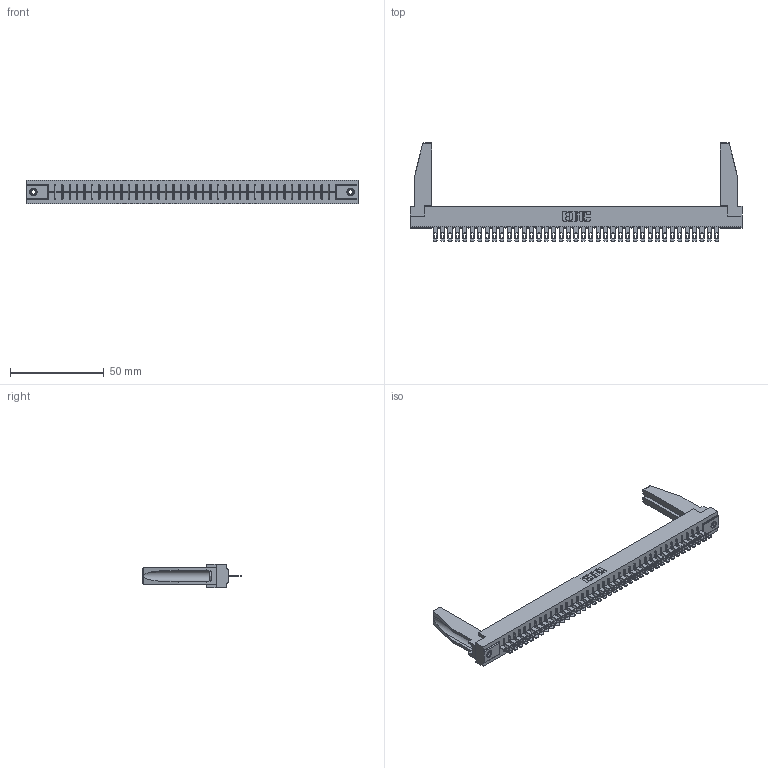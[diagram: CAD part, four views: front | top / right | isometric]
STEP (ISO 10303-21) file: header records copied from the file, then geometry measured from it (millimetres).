
FILE_DESCRIPTION (( 'STEP AP203' ), '1' );
FILE_NAME ('356-039-400-178.STEP', '2020-09-24T00:03:07', ( '' ), ( '' ), 'SwSTEP 2.0', 'SolidWorks 2020', '' );
FILE_SCHEMA (( 'CONFIG_CONTROL_DESIGN' ));
Length unit declared in the file: inch
Products named in the file (5): 306 Part_.156 Dia; 356-039-400-178; 307-220-078; 306-290-001_100; 345-250-001_345-250-001-102
Assembly tree (44 placements, depth 2):
  356-039-400-178
    306 Part_.156 Dia
    306-290-001_100  x39
    345-250-001_345-250-001-102  x2
    307-220-078  x2
Bounding box: 177.55 x 52.91 x 12.7 mm (x, y, z)
Volume: 23725.5 mm3; surface area: 24741.1 mm2
Topology: 44 solids, 44 shells, 3210 faces, 9031 edges, 5802 vertices
Faces by surface type: plane 2102, cylinder 936, sphere 156, cone 12, torus 4
Entity records: 39361 total; most frequent: CARTESIAN_POINT 6610, ORIENTED_EDGE 6512, DIRECTION 6470, EDGE_CURVE 3256, VECTOR 2546, LINE 2546, VERTEX_POINT 2060, AXIS2_PLACEMENT_3D 1962
